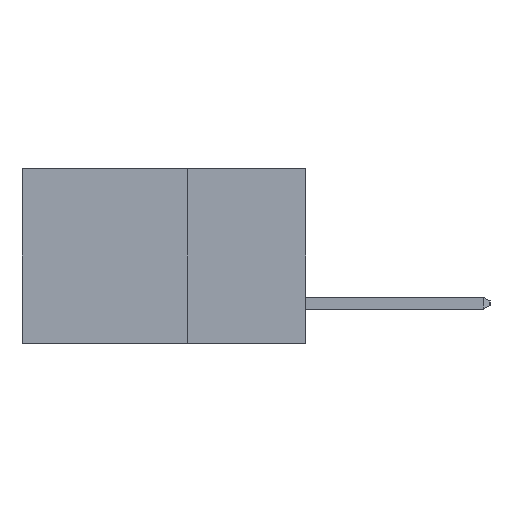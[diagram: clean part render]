
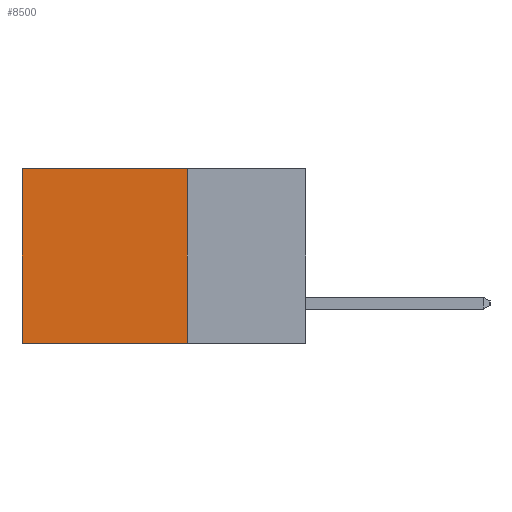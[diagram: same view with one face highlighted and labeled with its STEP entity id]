
A CAD part, left-side view. The second image highlights one B-rep face of the part: STEP entity #8500.
In plain terms, the highlighted planar face has unit normal (-1, 0, 0).
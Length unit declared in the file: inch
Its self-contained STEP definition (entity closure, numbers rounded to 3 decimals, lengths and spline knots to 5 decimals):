
#903 = LINE ( 'NONE', #18887, #5095 ) ;
#1035 = CARTESIAN_POINT ( 'NONE',  ( 0.298, 0.6, 0. ) ) ;
#1713 = ORIENTED_EDGE ( 'NONE', *, *, #10424, .T. ) ;
#2437 = VECTOR ( 'NONE', #14844, 39.37008 ) ;
#2580 = ORIENTED_EDGE ( 'NONE', *, *, #12266, .F. ) ;
#3203 = ORIENTED_EDGE ( 'NONE', *, *, #11456, .F. ) ;
#3429 = LINE ( 'NONE', #1035, #2437 ) ;
#3438 = VERTEX_POINT ( 'NONE', #9521 ) ;
#3487 = FACE_OUTER_BOUND ( 'NONE', #9501, .T. ) ;
#4266 = ORIENTED_EDGE ( 'NONE', *, *, #15766, .T. ) ;
#4926 = DIRECTION ( 'NONE',  ( 0., 0., -1. ) ) ;
#5095 = VECTOR ( 'NONE', #5502, 39.37008 ) ;
#5502 = DIRECTION ( 'NONE',  ( 0., 0., -1. ) ) ;
#7247 = DIRECTION ( 'NONE',  ( 0., 1., 0. ) ) ;
#7756 = VECTOR ( 'NONE', #14086, 39.37008 ) ;
#8500 = ADVANCED_FACE ( 'NONE', ( #3487 ), #10970, .F. ) ;
#9501 = EDGE_LOOP ( 'NONE', ( #1713, #3203, #2580, #4266 ) ) ;
#9521 = CARTESIAN_POINT ( 'NONE',  ( 0.298, 0.6, -0.37 ) ) ;
#9827 = VERTEX_POINT ( 'NONE', #11975 ) ;
#10253 = LINE ( 'NONE', #17746, #13813 ) ;
#10424 = EDGE_CURVE ( 'NONE', #13710, #3438, #3429, .T. ) ;
#10970 = PLANE ( 'NONE',  #15186 ) ;
#11456 = EDGE_CURVE ( 'NONE', #9827, #3438, #16718, .T. ) ;
#11975 = CARTESIAN_POINT ( 'NONE',  ( 0.298, 0.25, -0.37 ) ) ;
#12266 = EDGE_CURVE ( 'NONE', #17068, #9827, #903, .T. ) ;
#13710 = VERTEX_POINT ( 'NONE', #16730 ) ;
#13813 = VECTOR ( 'NONE', #7247, 39.37008 ) ;
#13944 = CARTESIAN_POINT ( 'NONE',  ( 0.298, 0.25, 0. ) ) ;
#14008 = DIRECTION ( 'NONE',  ( 1., 0., 0. ) ) ;
#14086 = DIRECTION ( 'NONE',  ( 0., 1., 0. ) ) ;
#14844 = DIRECTION ( 'NONE',  ( 0., 0., -1. ) ) ;
#15186 = AXIS2_PLACEMENT_3D ( 'NONE', #13944, #14008, #4926 ) ;
#15766 = EDGE_CURVE ( 'NONE', #17068, #13710, #10253, .T. ) ;
#16379 = CARTESIAN_POINT ( 'NONE',  ( 0.298, 0.25, 0. ) ) ;
#16718 = LINE ( 'NONE', #18491, #7756 ) ;
#16730 = CARTESIAN_POINT ( 'NONE',  ( 0.298, 0.6, 0. ) ) ;
#17068 = VERTEX_POINT ( 'NONE', #16379 ) ;
#17746 = CARTESIAN_POINT ( 'NONE',  ( 0.298, 0.25, 0. ) ) ;
#18491 = CARTESIAN_POINT ( 'NONE',  ( 0.298, 0.25, -0.37 ) ) ;
#18887 = CARTESIAN_POINT ( 'NONE',  ( 0.298, 0.25, 0. ) ) ;
